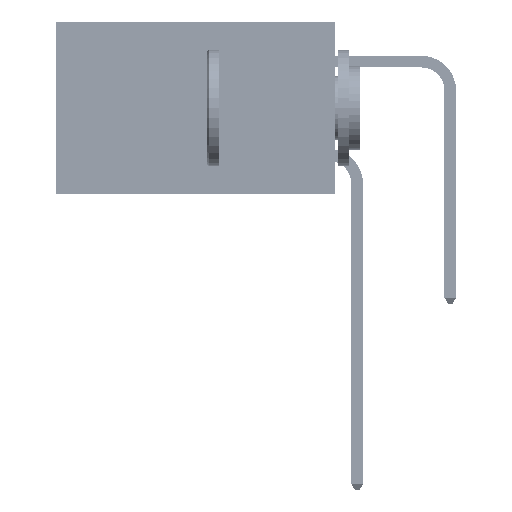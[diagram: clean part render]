
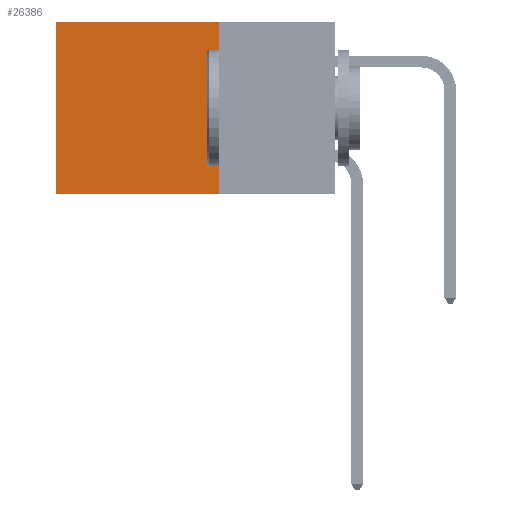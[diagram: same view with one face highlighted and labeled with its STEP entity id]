
A CAD part, left-side view. The second image highlights one B-rep face of the part: STEP entity #26386.
In plain terms, the highlighted planar face has unit normal (-1, 0, 0).
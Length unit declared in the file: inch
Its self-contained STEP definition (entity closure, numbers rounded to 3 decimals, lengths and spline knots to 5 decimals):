
#4231 = CARTESIAN_POINT ( 'NONE',  ( 0.2875, 0.25, -0.37 ) ) ;
#6648 = FACE_OUTER_BOUND ( 'NONE', #46805, .T. ) ;
#6838 = ORIENTED_EDGE ( 'NONE', *, *, #34886, .T. ) ;
#12266 = EDGE_CURVE ( 'NONE', #37860, #46698, #29501, .T. ) ;
#13954 = DIRECTION ( 'NONE',  ( 1., 0., 0. ) ) ;
#14151 = CARTESIAN_POINT ( 'NONE',  ( 0.2875, 0.25, 0. ) ) ;
#17970 = DIRECTION ( 'NONE',  ( 0., 0., -1. ) ) ;
#20159 = CARTESIAN_POINT ( 'NONE',  ( 0.2875, 0.6, 0. ) ) ;
#21648 = VERTEX_POINT ( 'NONE', #48311 ) ;
#22400 = LINE ( 'NONE', #20159, #24907 ) ;
#22643 = DIRECTION ( 'NONE',  ( 0., 1., 0. ) ) ;
#24090 = CARTESIAN_POINT ( 'NONE',  ( 0.2875, 0.6, -0.37 ) ) ;
#24303 = VECTOR ( 'NONE', #25678, 39.37008 ) ;
#24441 = DIRECTION ( 'NONE',  ( 0., 1., 0. ) ) ;
#24907 = VECTOR ( 'NONE', #40003, 39.37008 ) ;
#25231 = EDGE_CURVE ( 'NONE', #45055, #46698, #22400, .T. ) ;
#25678 = DIRECTION ( 'NONE',  ( 0., 0., -1. ) ) ;
#26386 = ADVANCED_FACE ( 'NONE', ( #6648 ), #49970, .F. ) ;
#26493 = CARTESIAN_POINT ( 'NONE',  ( 0.2875, 0.25, 0. ) ) ;
#29501 = LINE ( 'NONE', #4231, #40089 ) ;
#34086 = CARTESIAN_POINT ( 'NONE',  ( 0.2875, 0.25, -0.37 ) ) ;
#34843 = LINE ( 'NONE', #14151, #24303 ) ;
#34886 = EDGE_CURVE ( 'NONE', #21648, #45055, #50468, .T. ) ;
#37116 = ORIENTED_EDGE ( 'NONE', *, *, #12266, .F. ) ;
#37403 = VECTOR ( 'NONE', #22643, 39.37008 ) ;
#37550 = ORIENTED_EDGE ( 'NONE', *, *, #45264, .F. ) ;
#37860 = VERTEX_POINT ( 'NONE', #34086 ) ;
#40003 = DIRECTION ( 'NONE',  ( 0., 0., -1. ) ) ;
#40089 = VECTOR ( 'NONE', #24441, 39.37008 ) ;
#44163 = CARTESIAN_POINT ( 'NONE',  ( 0.2875, 0.6, 0. ) ) ;
#45055 = VERTEX_POINT ( 'NONE', #44163 ) ;
#45264 = EDGE_CURVE ( 'NONE', #21648, #37860, #34843, .T. ) ;
#46508 = CARTESIAN_POINT ( 'NONE',  ( 0.2875, 0.25, 0. ) ) ;
#46698 = VERTEX_POINT ( 'NONE', #24090 ) ;
#46805 = EDGE_LOOP ( 'NONE', ( #48917, #37116, #37550, #6838 ) ) ;
#48311 = CARTESIAN_POINT ( 'NONE',  ( 0.2875, 0.25, 0. ) ) ;
#48640 = AXIS2_PLACEMENT_3D ( 'NONE', #26493, #13954, #17970 ) ;
#48917 = ORIENTED_EDGE ( 'NONE', *, *, #25231, .T. ) ;
#49970 = PLANE ( 'NONE',  #48640 ) ;
#50468 = LINE ( 'NONE', #46508, #37403 ) ;
